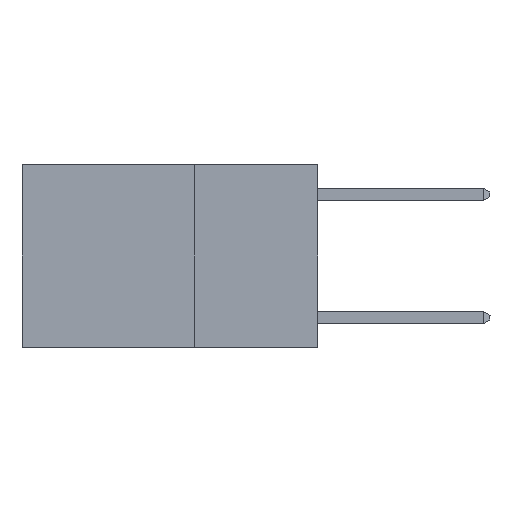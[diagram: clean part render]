
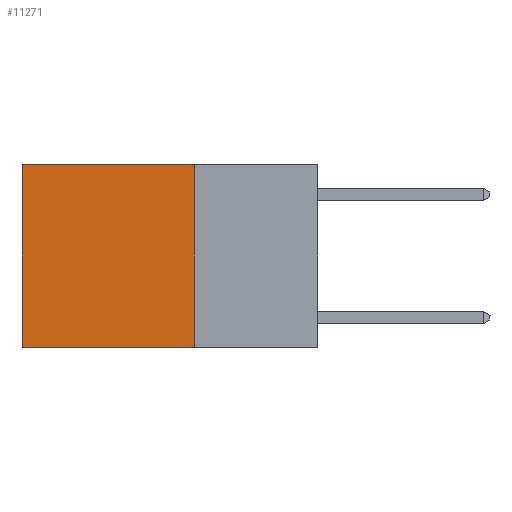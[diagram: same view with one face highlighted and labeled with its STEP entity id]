
A CAD part, left-side view. The second image highlights one B-rep face of the part: STEP entity #11271.
In plain terms, the highlighted planar face has unit normal (-1, 0, 0).
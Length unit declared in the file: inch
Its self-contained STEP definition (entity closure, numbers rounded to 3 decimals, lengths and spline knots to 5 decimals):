
#487 = CARTESIAN_POINT ( 'NONE',  ( 0.2625, 0.6, 0. ) ) ;
#889 = CARTESIAN_POINT ( 'NONE',  ( 0.2625, 0.25, 0. ) ) ;
#1184 = EDGE_CURVE ( 'NONE', #10511, #10964, #8547, .T. ) ;
#1618 = CARTESIAN_POINT ( 'NONE',  ( 0.2625, 0.25, -0.37 ) ) ;
#1705 = LINE ( 'NONE', #889, #7215 ) ;
#1913 = ORIENTED_EDGE ( 'NONE', *, *, #6060, .F. ) ;
#2459 = LINE ( 'NONE', #7696, #9362 ) ;
#2605 = DIRECTION ( 'NONE',  ( 1., 0., 0. ) ) ;
#2919 = EDGE_CURVE ( 'NONE', #10964, #6066, #2459, .T. ) ;
#2956 = VERTEX_POINT ( 'NONE', #7562 ) ;
#3344 = EDGE_CURVE ( 'NONE', #10511, #2956, #1705, .T. ) ;
#3482 = DIRECTION ( 'NONE',  ( 0., 1., 0. ) ) ;
#3796 = AXIS2_PLACEMENT_3D ( 'NONE', #5280, #2605, #10892 ) ;
#4287 = VECTOR ( 'NONE', #7785, 39.37008 ) ;
#4825 = VECTOR ( 'NONE', #3482, 39.37008 ) ;
#4867 = ORIENTED_EDGE ( 'NONE', *, *, #1184, .T. ) ;
#5280 = CARTESIAN_POINT ( 'NONE',  ( 0.2625, 0.25, 0. ) ) ;
#6019 = CARTESIAN_POINT ( 'NONE',  ( 0.2625, 0.25, 0. ) ) ;
#6060 = EDGE_CURVE ( 'NONE', #2956, #6066, #8901, .T. ) ;
#6066 = VERTEX_POINT ( 'NONE', #10844 ) ;
#7215 = VECTOR ( 'NONE', #11003, 39.37008 ) ;
#7562 = CARTESIAN_POINT ( 'NONE',  ( 0.2625, 0.25, -0.37 ) ) ;
#7696 = CARTESIAN_POINT ( 'NONE',  ( 0.2625, 0.6, 0. ) ) ;
#7785 = DIRECTION ( 'NONE',  ( 0., 1., 0. ) ) ;
#8547 = LINE ( 'NONE', #6019, #4287 ) ;
#8901 = LINE ( 'NONE', #1618, #4825 ) ;
#8906 = ORIENTED_EDGE ( 'NONE', *, *, #2919, .T. ) ;
#9175 = PLANE ( 'NONE',  #3796 ) ;
#9257 = CARTESIAN_POINT ( 'NONE',  ( 0.2625, 0.25, 0. ) ) ;
#9362 = VECTOR ( 'NONE', #10279, 39.37008 ) ;
#9594 = EDGE_LOOP ( 'NONE', ( #8906, #1913, #10848, #4867 ) ) ;
#10279 = DIRECTION ( 'NONE',  ( 0., 0., -1. ) ) ;
#10511 = VERTEX_POINT ( 'NONE', #9257 ) ;
#10844 = CARTESIAN_POINT ( 'NONE',  ( 0.2625, 0.6, -0.37 ) ) ;
#10848 = ORIENTED_EDGE ( 'NONE', *, *, #3344, .F. ) ;
#10892 = DIRECTION ( 'NONE',  ( 0., 0., -1. ) ) ;
#10964 = VERTEX_POINT ( 'NONE', #487 ) ;
#11003 = DIRECTION ( 'NONE',  ( 0., 0., -1. ) ) ;
#11271 = ADVANCED_FACE ( 'NONE', ( #11729 ), #9175, .F. ) ;
#11729 = FACE_OUTER_BOUND ( 'NONE', #9594, .T. ) ;
